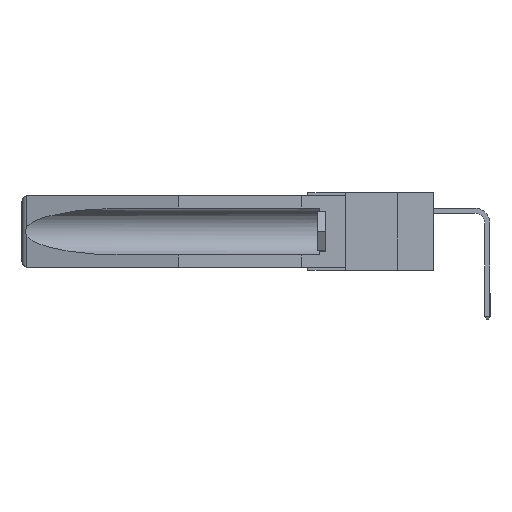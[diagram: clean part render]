
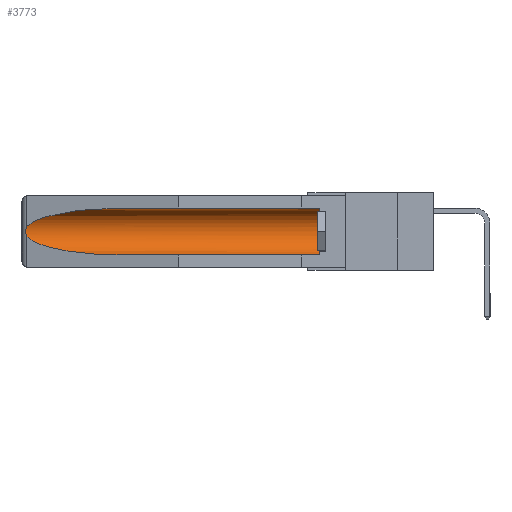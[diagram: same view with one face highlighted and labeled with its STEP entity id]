
A CAD part, left-side view. The second image highlights one B-rep face of the part: STEP entity #3773.
In plain terms, the highlighted cylindrical face has radius 2.857 mm (diameter 5.715 mm), a partial arc.
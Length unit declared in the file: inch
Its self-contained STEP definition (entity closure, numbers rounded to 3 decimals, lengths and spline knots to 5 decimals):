
#1068 = CARTESIAN_POINT ( 'NONE',  ( 0.2675, 1.53308, -0.16763 ) ) ;
#1424 = VERTEX_POINT ( 'NONE', #5643 ) ;
#1769 = DIRECTION ( 'NONE',  ( 0., 1., 0. ) ) ;
#2157 =( BOUNDED_CURVE ( )  B_SPLINE_CURVE ( 3, ( #5006, #12807, #19149, #9840 ),
 .UNSPECIFIED., .F., .F. ) 
 B_SPLINE_CURVE_WITH_KNOTS ( ( 4, 4 ),
 ( 4.71239, 6.08839 ),
 .UNSPECIFIED. ) 
 CURVE ( )  GEOMETRIC_REPRESENTATION_ITEM ( )  RATIONAL_B_SPLINE_CURVE ( ( 1., 0.848, 0.848, 1. ) ) 
 REPRESENTATION_ITEM ( '' )  );
#2268 = CARTESIAN_POINT ( 'NONE',  ( 0.155, 0.126, -0.059 ) ) ;
#2654 = CYLINDRICAL_SURFACE ( 'NONE', #17887, 0.1125 ) ;
#2727 = CARTESIAN_POINT ( 'NONE',  ( 0.2673, 1.53269, -0.17917 ) ) ;
#3246 = CARTESIAN_POINT ( 'NONE',  ( 0.155, 1.07973, -0.059 ) ) ;
#3504 = CARTESIAN_POINT ( 'NONE',  ( 0.26537, 1.52718, -0.19328 ) ) ;
#3773 = ADVANCED_FACE ( 'NONE', ( #19382 ), #2654, .F. ) ;
#4076 = ORIENTED_EDGE ( 'NONE', *, *, #10494, .T. ) ;
#4103 = CARTESIAN_POINT ( 'NONE',  ( 0.155, 1.07973, -0.284 ) ) ;
#4130 = CARTESIAN_POINT ( 'NONE',  ( 0.26655, 1.53094, -0.18657 ) ) ;
#4343 = EDGE_CURVE ( 'NONE', #11498, #6881, #14337, .T. ) ;
#4547 = VERTEX_POINT ( 'NONE', #3246 ) ;
#4967 = ORIENTED_EDGE ( 'NONE', *, *, #15803, .F. ) ;
#5006 = CARTESIAN_POINT ( 'NONE',  ( 0.155, 1.07973, -0.059 ) ) ;
#5220 = ORIENTED_EDGE ( 'NONE', *, *, #4343, .T. ) ;
#5643 = CARTESIAN_POINT ( 'NONE',  ( 0.155, 0.126, -0.284 ) ) ;
#5645 = CARTESIAN_POINT ( 'NONE',  ( 0.26537, 1.52718, -0.19328 ) ) ;
#5799 = CARTESIAN_POINT ( 'NONE',  ( 0.26537, 1.52718, -0.19328 ) ) ;
#6059 = DIRECTION ( 'NONE',  ( 0., 0., 1. ) ) ;
#6684 = VERTEX_POINT ( 'NONE', #2268 ) ;
#6688 = CARTESIAN_POINT ( 'NONE',  ( 0.155, -0.30754, -0.284 ) ) ;
#6797 = DIRECTION ( 'NONE',  ( 0., 1., 0. ) ) ;
#6881 = VERTEX_POINT ( 'NONE', #12275 ) ;
#7014 = LINE ( 'NONE', #6688, #7259 ) ;
#7259 = VECTOR ( 'NONE', #1769, 39.37008 ) ;
#8946 = CARTESIAN_POINT ( 'NONE',  ( 0.26537, 1.52718, -0.14972 ) ) ;
#9160 = LINE ( 'NONE', #15572, #16601 ) ;
#9253 = VERTEX_POINT ( 'NONE', #15010 ) ;
#9642 = ORIENTED_EDGE ( 'NONE', *, *, #11809, .T. ) ;
#9840 = CARTESIAN_POINT ( 'NONE',  ( 0.26537, 1.52718, -0.14972 ) ) ;
#10494 = EDGE_CURVE ( 'NONE', #6684, #4547, #9160, .T. ) ;
#10525 = CARTESIAN_POINT ( 'NONE',  ( 0.2675, 1.53308, -0.17534 ) ) ;
#10629 = DIRECTION ( 'NONE',  ( 0., -1., 0. ) ) ;
#11498 = VERTEX_POINT ( 'NONE', #3504 ) ;
#11809 = EDGE_CURVE ( 'NONE', #9253, #11498, #14605, .T. ) ;
#11929 = CARTESIAN_POINT ( 'NONE',  ( 0.26654, 1.53092, -0.15636 ) ) ;
#12275 = CARTESIAN_POINT ( 'NONE',  ( 0.155, 1.07973, -0.284 ) ) ;
#12807 = CARTESIAN_POINT ( 'NONE',  ( 0.21114, 1.30732, -0.059 ) ) ;
#13457 = EDGE_CURVE ( 'NONE', #1424, #6684, #14419, .T. ) ;
#13530 = CARTESIAN_POINT ( 'NONE',  ( 0.25451, 1.48313, -0.24835 ) ) ;
#13702 = CARTESIAN_POINT ( 'NONE',  ( 0.26597, 1.5296, -0.19026 ) ) ;
#14279 = EDGE_CURVE ( 'NONE', #4547, #9253, #2157, .T. ) ;
#14337 =( BOUNDED_CURVE ( )  B_SPLINE_CURVE ( 3, ( #5799, #13530, #15172, #4103 ),
 .UNSPECIFIED., .F., .F. ) 
 B_SPLINE_CURVE_WITH_KNOTS ( ( 4, 4 ),
 ( 0.1948, 1.5708 ),
 .UNSPECIFIED. ) 
 CURVE ( )  GEOMETRIC_REPRESENTATION_ITEM ( )  RATIONAL_B_SPLINE_CURVE ( ( 1., 0.848, 0.848, 1. ) ) 
 REPRESENTATION_ITEM ( '' )  );
#14419 = CIRCLE ( 'NONE', #16998, 0.1125 ) ;
#14605 = B_SPLINE_CURVE_WITH_KNOTS ( 'NONE', 3,
 ( #8946, #19986, #11929, #16757, #1068, #10525, #2727, #4130, #13702, #5645 ),
 .UNSPECIFIED., .F., .F.,
 ( 4, 2, 2, 2, 4 ),
 ( 0., 0.00029, 0.00058, 0.00087, 0.00117 ),
 .UNSPECIFIED. ) ;
#14783 = CARTESIAN_POINT ( 'NONE',  ( 0.155, -0.30754, -0.1715 ) ) ;
#15010 = CARTESIAN_POINT ( 'NONE',  ( 0.26537, 1.52718, -0.14972 ) ) ;
#15172 = CARTESIAN_POINT ( 'NONE',  ( 0.21114, 1.30732, -0.284 ) ) ;
#15572 = CARTESIAN_POINT ( 'NONE',  ( 0.155, -0.30754, -0.059 ) ) ;
#15803 = EDGE_CURVE ( 'NONE', #1424, #6881, #7014, .T. ) ;
#16579 = ORIENTED_EDGE ( 'NONE', *, *, #14279, .T. ) ;
#16601 = VECTOR ( 'NONE', #18790, 39.37008 ) ;
#16757 = CARTESIAN_POINT ( 'NONE',  ( 0.2673, 1.5327, -0.16383 ) ) ;
#16998 = AXIS2_PLACEMENT_3D ( 'NONE', #18545, #10629, #6059 ) ;
#17887 = AXIS2_PLACEMENT_3D ( 'NONE', #14783, #6797, #20002 ) ;
#18450 = ORIENTED_EDGE ( 'NONE', *, *, #13457, .T. ) ;
#18545 = CARTESIAN_POINT ( 'NONE',  ( 0.155, 0.126, -0.1715 ) ) ;
#18790 = DIRECTION ( 'NONE',  ( 0., 1., 0. ) ) ;
#19099 = EDGE_LOOP ( 'NONE', ( #16579, #9642, #5220, #4967, #18450, #4076 ) ) ;
#19149 = CARTESIAN_POINT ( 'NONE',  ( 0.25451, 1.48313, -0.09465 ) ) ;
#19382 = FACE_OUTER_BOUND ( 'NONE', #19099, .T. ) ;
#19986 = CARTESIAN_POINT ( 'NONE',  ( 0.26597, 1.52961, -0.15275 ) ) ;
#20002 = DIRECTION ( 'NONE',  ( 0., 0., 1. ) ) ;
